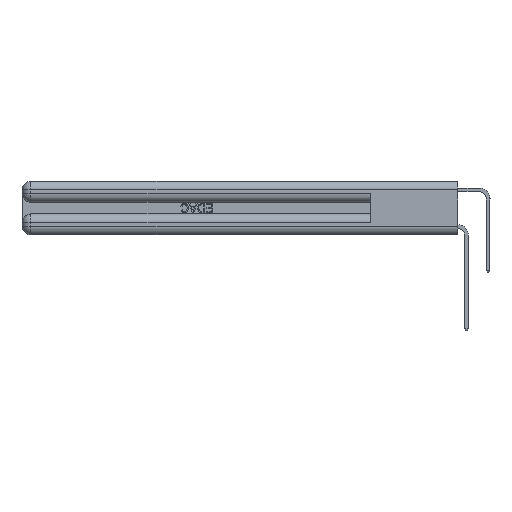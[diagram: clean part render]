
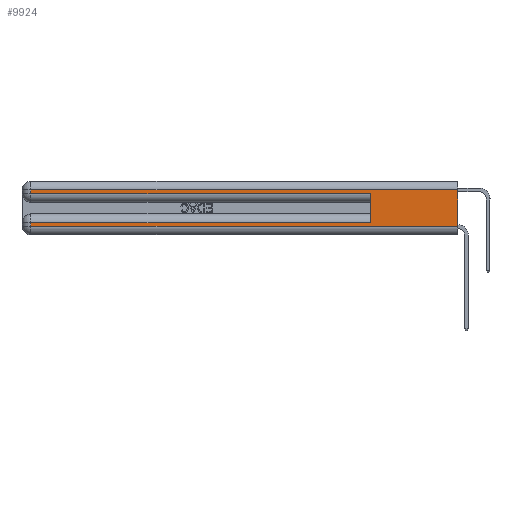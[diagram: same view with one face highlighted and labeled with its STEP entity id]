
A CAD part, left-side view. The second image highlights one B-rep face of the part: STEP entity #9924.
In plain terms, the highlighted planar face has unit normal (-1, 0, 0).
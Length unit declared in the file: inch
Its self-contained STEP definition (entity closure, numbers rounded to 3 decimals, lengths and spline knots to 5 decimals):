
#356 = VERTEX_POINT ( 'NONE', #26695 ) ;
#998 = DIRECTION ( 'NONE',  ( 0., 0., -1. ) ) ;
#2192 = CARTESIAN_POINT ( 'NONE',  ( 0., 2.94, 0.285 ) ) ;
#2213 = DIRECTION ( 'NONE',  ( 0., -1., 0. ) ) ;
#2248 = EDGE_CURVE ( 'NONE', #26430, #13621, #4067, .T. ) ;
#2694 = DIRECTION ( 'NONE',  ( 0., 1., 0. ) ) ;
#3415 = ORIENTED_EDGE ( 'NONE', *, *, #3735, .T. ) ;
#3735 = EDGE_CURVE ( 'NONE', #24817, #33992, #13214, .T. ) ;
#4002 = FACE_OUTER_BOUND ( 'NONE', #15106, .T. ) ;
#4067 = LINE ( 'NONE', #5385, #25214 ) ;
#4671 = ORIENTED_EDGE ( 'NONE', *, *, #33753, .T. ) ;
#5385 = CARTESIAN_POINT ( 'NONE',  ( 0., 0., 0.31 ) ) ;
#5486 = LINE ( 'NONE', #8619, #27492 ) ;
#5620 = CARTESIAN_POINT ( 'NONE',  ( 0., 0., 0.31 ) ) ;
#6028 = CARTESIAN_POINT ( 'NONE',  ( 0., 2.94, 0.06 ) ) ;
#6126 = EDGE_CURVE ( 'NONE', #20453, #24817, #31778, .T. ) ;
#6498 = VECTOR ( 'NONE', #2213, 39.37008 ) ;
#6784 = DIRECTION ( 'NONE',  ( 0., 0., -1. ) ) ;
#6867 = CARTESIAN_POINT ( 'NONE',  ( 0., 2.94, 0.37 ) ) ;
#7105 = ORIENTED_EDGE ( 'NONE', *, *, #12503, .T. ) ;
#7170 = EDGE_CURVE ( 'NONE', #13621, #27115, #5486, .T. ) ;
#8307 = CARTESIAN_POINT ( 'NONE',  ( 0., 2.94, 0.31 ) ) ;
#8416 = PLANE ( 'NONE',  #26150 ) ;
#8430 = VECTOR ( 'NONE', #25867, 39.37008 ) ;
#8500 = ORIENTED_EDGE ( 'NONE', *, *, #18924, .F. ) ;
#8619 = CARTESIAN_POINT ( 'NONE',  ( 0., 2.94, 0.37 ) ) ;
#9459 = CARTESIAN_POINT ( 'NONE',  ( 0., 0., 0.37 ) ) ;
#9478 = CARTESIAN_POINT ( 'NONE',  ( 0., 0., 0.06 ) ) ;
#9681 = VECTOR ( 'NONE', #2694, 39.37008 ) ;
#9817 = ORIENTED_EDGE ( 'NONE', *, *, #2248, .T. ) ;
#9924 = ADVANCED_FACE ( 'NONE', ( #4002 ), #8416, .F. ) ;
#11101 = VECTOR ( 'NONE', #22711, 39.37008 ) ;
#11330 = DIRECTION ( 'NONE',  ( 0., 0., -1. ) ) ;
#11973 = ORIENTED_EDGE ( 'NONE', *, *, #6126, .T. ) ;
#12503 = EDGE_CURVE ( 'NONE', #27115, #34824, #20050, .T. ) ;
#13214 = LINE ( 'NONE', #25469, #11101 ) ;
#13394 = CARTESIAN_POINT ( 'NONE',  ( 0., 0., 0.085 ) ) ;
#13621 = VERTEX_POINT ( 'NONE', #8307 ) ;
#14264 = DIRECTION ( 'NONE',  ( 0., 1., 0. ) ) ;
#14331 = LINE ( 'NONE', #20032, #16889 ) ;
#14562 = LINE ( 'NONE', #17173, #17961 ) ;
#15106 = EDGE_LOOP ( 'NONE', ( #17892, #9817, #16662, #7105, #8500, #4671, #11973, #3415 ) ) ;
#16662 = ORIENTED_EDGE ( 'NONE', *, *, #7170, .T. ) ;
#16889 = VECTOR ( 'NONE', #6784, 39.37008 ) ;
#17173 = CARTESIAN_POINT ( 'NONE',  ( 0., 0.6, 0.145 ) ) ;
#17892 = ORIENTED_EDGE ( 'NONE', *, *, #22917, .F. ) ;
#17905 = CARTESIAN_POINT ( 'NONE',  ( 0., 0.6, 0.285 ) ) ;
#17961 = VECTOR ( 'NONE', #22655, 39.37008 ) ;
#18924 = EDGE_CURVE ( 'NONE', #356, #34824, #14562, .T. ) ;
#20032 = CARTESIAN_POINT ( 'NONE',  ( 0., 0., 0.37 ) ) ;
#20050 = LINE ( 'NONE', #23743, #6498 ) ;
#20453 = VERTEX_POINT ( 'NONE', #20521 ) ;
#20521 = CARTESIAN_POINT ( 'NONE',  ( 0., 2.94, 0.085 ) ) ;
#22655 = DIRECTION ( 'NONE',  ( 0., 0., 1. ) ) ;
#22711 = DIRECTION ( 'NONE',  ( 0., -1., 0. ) ) ;
#22917 = EDGE_CURVE ( 'NONE', #26430, #33992, #14331, .T. ) ;
#23743 = CARTESIAN_POINT ( 'NONE',  ( 0., 0., 0.285 ) ) ;
#24817 = VERTEX_POINT ( 'NONE', #6028 ) ;
#25214 = VECTOR ( 'NONE', #14264, 39.37008 ) ;
#25469 = CARTESIAN_POINT ( 'NONE',  ( 0., 0., 0.06 ) ) ;
#25867 = DIRECTION ( 'NONE',  ( 0., 0., -1. ) ) ;
#26150 = AXIS2_PLACEMENT_3D ( 'NONE', #9459, #33477, #998 ) ;
#26430 = VERTEX_POINT ( 'NONE', #5620 ) ;
#26695 = CARTESIAN_POINT ( 'NONE',  ( 0., 0.6, 0.085 ) ) ;
#27115 = VERTEX_POINT ( 'NONE', #2192 ) ;
#27492 = VECTOR ( 'NONE', #11330, 39.37008 ) ;
#29171 = LINE ( 'NONE', #13394, #9681 ) ;
#31778 = LINE ( 'NONE', #6867, #8430 ) ;
#33477 = DIRECTION ( 'NONE',  ( 1., 0., 0. ) ) ;
#33753 = EDGE_CURVE ( 'NONE', #356, #20453, #29171, .T. ) ;
#33992 = VERTEX_POINT ( 'NONE', #9478 ) ;
#34824 = VERTEX_POINT ( 'NONE', #17905 ) ;
